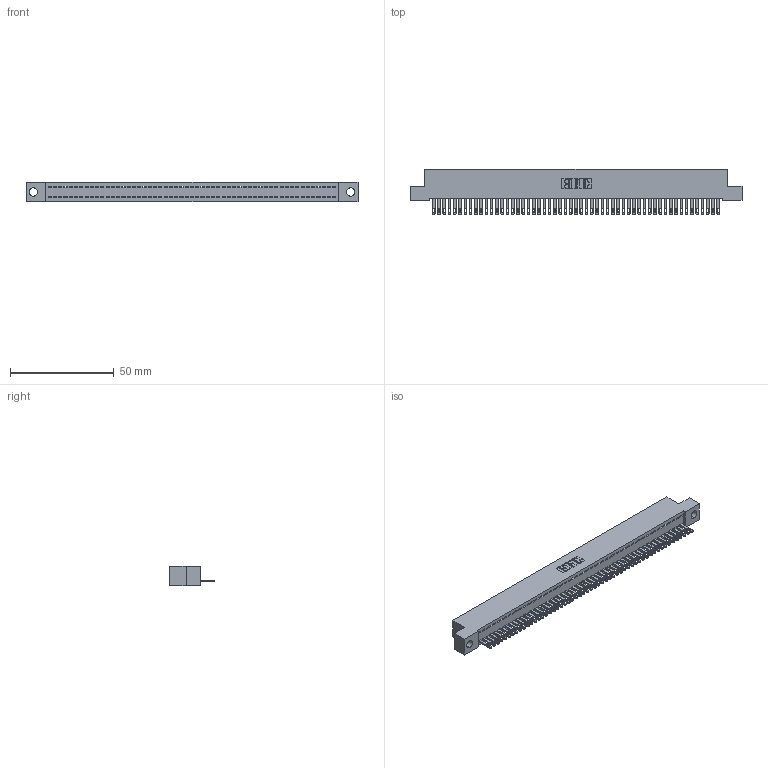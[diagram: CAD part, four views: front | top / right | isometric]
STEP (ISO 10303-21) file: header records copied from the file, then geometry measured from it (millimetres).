
FILE_DESCRIPTION (( 'STEP AP203' ), '1' );
FILE_NAME ('892-055-500-104.STEP', '2020-09-21T18:32:34', ( '' ), ( '' ), 'SwSTEP 2.0', 'SolidWorks 2020', '' );
FILE_SCHEMA (( 'CONFIG_CONTROL_DESIGN' ));
Length unit declared in the file: inch
Products named in the file (3): 842 Part_.156 TH; 892-055-500-104; 345-292-001_345-293-100
Assembly tree (56 placements, depth 2):
  892-055-500-104
    842 Part_.156 TH
    345-292-001_345-293-100  x55
Bounding box: 160.02 x 21.85 x 9.4 mm (x, y, z)
Volume: 14025.5 mm3; surface area: 20765.5 mm2
Topology: 56 solids, 56 shells, 3080 faces, 9539 edges, 6358 vertices
Faces by surface type: plane 2046, cylinder 1034
Entity records: 31743 total; most frequent: CARTESIAN_POINT 5479, ORIENTED_EDGE 5470, DIRECTION 4597, EDGE_CURVE 2735, VECTOR 2603, LINE 2603, VERTEX_POINT 1822, AXIS2_PLACEMENT_3D 997
